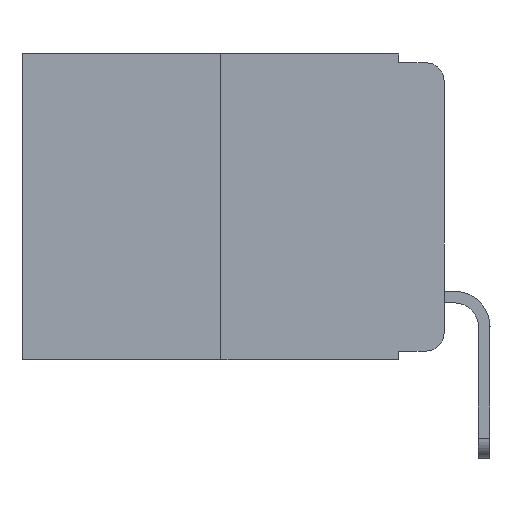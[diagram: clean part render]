
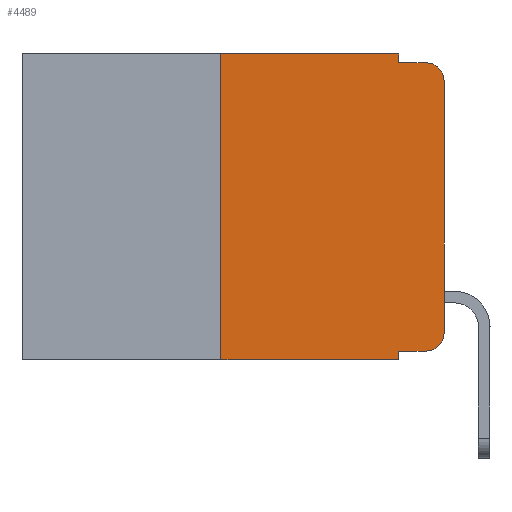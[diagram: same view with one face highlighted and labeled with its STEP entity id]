
A CAD part, left-side view. The second image highlights one B-rep face of the part: STEP entity #4489.
In plain terms, the highlighted planar face has unit normal (-1, 0, 0).
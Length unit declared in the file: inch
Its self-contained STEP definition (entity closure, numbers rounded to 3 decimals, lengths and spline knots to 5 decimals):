
#107 = LINE ( 'NONE', #7492, #2735 ) ;
#199 = ORIENTED_EDGE ( 'NONE', *, *, #9352, .F. ) ;
#200 = VECTOR ( 'NONE', #10105, 39.37008 ) ;
#307 = DIRECTION ( 'NONE',  ( 0., -1., 0. ) ) ;
#388 = CARTESIAN_POINT ( 'NONE',  ( 0., 0.02, -0.01 ) ) ;
#427 = EDGE_LOOP ( 'NONE', ( #778, #8679, #199, #9499, #7233, #2517, #1832, #961, #1741, #8167 ) ) ;
#468 = VERTEX_POINT ( 'NONE', #10161 ) ;
#519 = DIRECTION ( 'NONE',  ( 0., 0., -1. ) ) ;
#537 = LINE ( 'NONE', #7727, #6774 ) ;
#778 = ORIENTED_EDGE ( 'NONE', *, *, #8860, .T. ) ;
#847 = CARTESIAN_POINT ( 'NONE',  ( 0., 0.25, -0.343 ) ) ;
#954 = CARTESIAN_POINT ( 'NONE',  ( 0., 0.051, 0. ) ) ;
#961 = ORIENTED_EDGE ( 'NONE', *, *, #3183, .F. ) ;
#1099 = CARTESIAN_POINT ( 'NONE',  ( 0., 0.25, 0. ) ) ;
#1152 = CARTESIAN_POINT ( 'NONE',  ( 0., 0.473, -0.343 ) ) ;
#1181 = LINE ( 'NONE', #7759, #5945 ) ;
#1483 = LINE ( 'NONE', #7190, #7364 ) ;
#1741 = ORIENTED_EDGE ( 'NONE', *, *, #7909, .T. ) ;
#1832 = ORIENTED_EDGE ( 'NONE', *, *, #7853, .T. ) ;
#1874 = DIRECTION ( 'NONE',  ( 0., 0., 1. ) ) ;
#1941 = AXIS2_PLACEMENT_3D ( 'NONE', #4613, #6148, #9388 ) ;
#1955 = AXIS2_PLACEMENT_3D ( 'NONE', #8185, #3018, #8875 ) ;
#2063 = VECTOR ( 'NONE', #9804, 39.37008 ) ;
#2463 = LINE ( 'NONE', #4262, #5281 ) ;
#2517 = ORIENTED_EDGE ( 'NONE', *, *, #8804, .F. ) ;
#2585 = VERTEX_POINT ( 'NONE', #10055 ) ;
#2714 = EDGE_CURVE ( 'NONE', #3916, #5981, #5508, .T. ) ;
#2735 = VECTOR ( 'NONE', #6688, 39.37008 ) ;
#2787 = DIRECTION ( 'NONE',  ( 0., -1., 0. ) ) ;
#3018 = DIRECTION ( 'NONE',  ( -1., 0., 0. ) ) ;
#3183 = EDGE_CURVE ( 'NONE', #3214, #9046, #8159, .T. ) ;
#3214 = VERTEX_POINT ( 'NONE', #8208 ) ;
#3626 = EDGE_CURVE ( 'NONE', #9796, #8133, #1483, .T. ) ;
#3916 = VERTEX_POINT ( 'NONE', #8460 ) ;
#4005 = EDGE_CURVE ( 'NONE', #468, #2585, #8028, .T. ) ;
#4060 = DIRECTION ( 'NONE',  ( 0., 0., -1. ) ) ;
#4262 = CARTESIAN_POINT ( 'NONE',  ( 0., 0., 0. ) ) ;
#4489 = ADVANCED_FACE ( 'NONE', ( #8641 ), #8480, .F. ) ;
#4525 = DIRECTION ( 'NONE',  ( -1., 0., 0. ) ) ;
#4613 = CARTESIAN_POINT ( 'NONE',  ( 0., 0.473, 0. ) ) ;
#5240 = CARTESIAN_POINT ( 'NONE',  ( 0., 0.051, -0.01 ) ) ;
#5281 = VECTOR ( 'NONE', #1874, 39.37008 ) ;
#5508 = CIRCLE ( 'NONE', #1955, 0.02 ) ;
#5945 = VECTOR ( 'NONE', #307, 39.37008 ) ;
#5981 = VERTEX_POINT ( 'NONE', #388 ) ;
#6148 = DIRECTION ( 'NONE',  ( 1., 0., 0. ) ) ;
#6215 = CARTESIAN_POINT ( 'NONE',  ( 0., 0.02, -0.313 ) ) ;
#6688 = DIRECTION ( 'NONE',  ( 0., 0., 1. ) ) ;
#6774 = VECTOR ( 'NONE', #8461, 39.37008 ) ;
#6831 = AXIS2_PLACEMENT_3D ( 'NONE', #6215, #4525, #519 ) ;
#7062 = CARTESIAN_POINT ( 'NONE',  ( 0., 0.051, -0.343 ) ) ;
#7184 = VERTEX_POINT ( 'NONE', #847 ) ;
#7190 = CARTESIAN_POINT ( 'NONE',  ( 0., 0.051, 0. ) ) ;
#7233 = ORIENTED_EDGE ( 'NONE', *, *, #8622, .F. ) ;
#7281 = VECTOR ( 'NONE', #2787, 39.37008 ) ;
#7364 = VECTOR ( 'NONE', #4060, 39.37008 ) ;
#7492 = CARTESIAN_POINT ( 'NONE',  ( 0., 0.25, 0. ) ) ;
#7727 = CARTESIAN_POINT ( 'NONE',  ( 0., 0.473, 0. ) ) ;
#7759 = CARTESIAN_POINT ( 'NONE',  ( 0., 0.051, -0.01 ) ) ;
#7853 = EDGE_CURVE ( 'NONE', #7184, #9046, #8409, .T. ) ;
#7909 = EDGE_CURVE ( 'NONE', #3214, #468, #9428, .T. ) ;
#8028 = CIRCLE ( 'NONE', #6831, 0.02 ) ;
#8133 = VERTEX_POINT ( 'NONE', #5240 ) ;
#8159 = LINE ( 'NONE', #954, #2063 ) ;
#8167 = ORIENTED_EDGE ( 'NONE', *, *, #4005, .T. ) ;
#8185 = CARTESIAN_POINT ( 'NONE',  ( 0., 0.02, -0.03 ) ) ;
#8208 = CARTESIAN_POINT ( 'NONE',  ( 0., 0.051, -0.333 ) ) ;
#8392 = VERTEX_POINT ( 'NONE', #1099 ) ;
#8409 = LINE ( 'NONE', #1152, #7281 ) ;
#8460 = CARTESIAN_POINT ( 'NONE',  ( 0., 0., -0.03 ) ) ;
#8461 = DIRECTION ( 'NONE',  ( 0., -1., 0. ) ) ;
#8480 = PLANE ( 'NONE',  #1941 ) ;
#8524 = CARTESIAN_POINT ( 'NONE',  ( 0., 0.051, 0. ) ) ;
#8622 = EDGE_CURVE ( 'NONE', #8392, #9796, #537, .T. ) ;
#8641 = FACE_OUTER_BOUND ( 'NONE', #427, .T. ) ;
#8679 = ORIENTED_EDGE ( 'NONE', *, *, #2714, .T. ) ;
#8804 = EDGE_CURVE ( 'NONE', #7184, #8392, #107, .T. ) ;
#8860 = EDGE_CURVE ( 'NONE', #2585, #3916, #2463, .T. ) ;
#8875 = DIRECTION ( 'NONE',  ( 0., 0., -1. ) ) ;
#9046 = VERTEX_POINT ( 'NONE', #7062 ) ;
#9308 = CARTESIAN_POINT ( 'NONE',  ( 0., 0.051, -0.333 ) ) ;
#9352 = EDGE_CURVE ( 'NONE', #8133, #5981, #1181, .T. ) ;
#9388 = DIRECTION ( 'NONE',  ( 0., 0., -1. ) ) ;
#9428 = LINE ( 'NONE', #9308, #200 ) ;
#9499 = ORIENTED_EDGE ( 'NONE', *, *, #3626, .F. ) ;
#9796 = VERTEX_POINT ( 'NONE', #8524 ) ;
#9804 = DIRECTION ( 'NONE',  ( 0., 0., -1. ) ) ;
#10055 = CARTESIAN_POINT ( 'NONE',  ( 0., 0., -0.313 ) ) ;
#10105 = DIRECTION ( 'NONE',  ( 0., -1., 0. ) ) ;
#10161 = CARTESIAN_POINT ( 'NONE',  ( 0., 0.02, -0.333 ) ) ;
